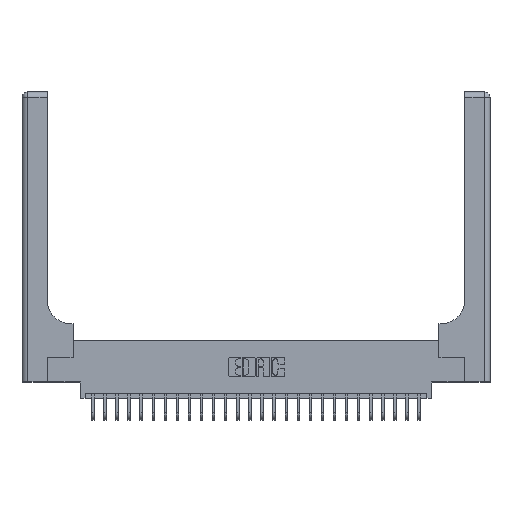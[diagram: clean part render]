
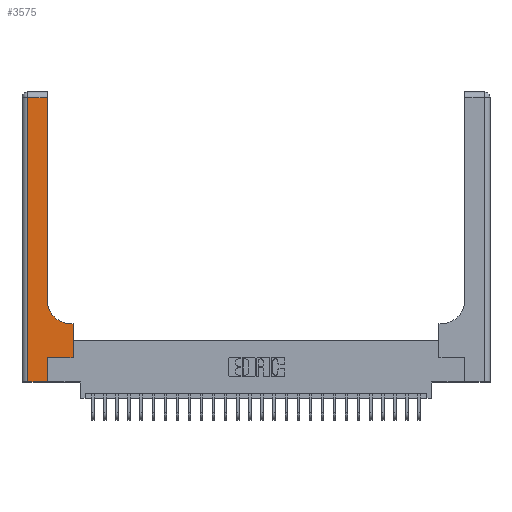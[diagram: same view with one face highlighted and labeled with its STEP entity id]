
A CAD part, top view. The second image highlights one B-rep face of the part: STEP entity #3575.
In plain terms, the highlighted planar face has unit normal (0, 0, 1).
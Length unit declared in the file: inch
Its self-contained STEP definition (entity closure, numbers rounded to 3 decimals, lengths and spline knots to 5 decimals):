
#247 = VERTEX_POINT ( 'NONE', #12926 ) ;
#473 = CARTESIAN_POINT ( 'NONE',  ( 0., 3., 0.37 ) ) ;
#620 = EDGE_CURVE ( 'NONE', #6042, #247, #7801, .T. ) ;
#866 = CARTESIAN_POINT ( 'NONE',  ( 0.06, 0., 0.37 ) ) ;
#962 = DIRECTION ( 'NONE',  ( -1., 0., 0. ) ) ;
#1192 = CARTESIAN_POINT ( 'NONE',  ( 0.265, 0.25, 0.37 ) ) ;
#1237 = EDGE_CURVE ( 'NONE', #19459, #6042, #15908, .T. ) ;
#1306 = DIRECTION ( 'NONE',  ( 0., 1., 0. ) ) ;
#1980 = EDGE_CURVE ( 'NONE', #247, #21757, #3933, .T. ) ;
#2104 = DIRECTION ( 'NONE',  ( -1., 0., 0. ) ) ;
#2456 = CARTESIAN_POINT ( 'NONE',  ( 0., 2.94, 0.37 ) ) ;
#2571 = CARTESIAN_POINT ( 'NONE',  ( 0.528, 0.25, 0.37 ) ) ;
#3368 = CARTESIAN_POINT ( 'NONE',  ( 0.26, 0.85, 0.37 ) ) ;
#3378 = CARTESIAN_POINT ( 'NONE',  ( 0.26, 3., 0.37 ) ) ;
#3511 = ORIENTED_EDGE ( 'NONE', *, *, #12563, .T. ) ;
#3575 = ADVANCED_FACE ( 'NONE', ( #25442 ), #13136, .F. ) ;
#3933 = LINE ( 'NONE', #5241, #25619 ) ;
#4005 = DIRECTION ( 'NONE',  ( 1., 0., 0. ) ) ;
#4239 = LINE ( 'NONE', #24141, #20331 ) ;
#4367 = VECTOR ( 'NONE', #2104, 39.37008 ) ;
#4563 = VERTEX_POINT ( 'NONE', #16521 ) ;
#4620 = CARTESIAN_POINT ( 'NONE',  ( 0.06, 3., 0.37 ) ) ;
#4726 = ORIENTED_EDGE ( 'NONE', *, *, #8363, .T. ) ;
#4866 = DIRECTION ( 'NONE',  ( -1., 0., 0. ) ) ;
#4985 = LINE ( 'NONE', #3378, #26697 ) ;
#5241 = CARTESIAN_POINT ( 'NONE',  ( 0.26, 0.6, 0.37 ) ) ;
#5452 = CIRCLE ( 'NONE', #27289, 0.25 ) ;
#6042 = VERTEX_POINT ( 'NONE', #22230 ) ;
#6170 = EDGE_CURVE ( 'NONE', #21757, #24052, #5452, .T. ) ;
#6517 = CARTESIAN_POINT ( 'NONE',  ( 0.265, 0.25, 0.37 ) ) ;
#7495 = VECTOR ( 'NONE', #4005, 39.37008 ) ;
#7801 = LINE ( 'NONE', #2571, #16007 ) ;
#8273 = ORIENTED_EDGE ( 'NONE', *, *, #1980, .T. ) ;
#8363 = EDGE_CURVE ( 'NONE', #4563, #13589, #18525, .T. ) ;
#8465 = ORIENTED_EDGE ( 'NONE', *, *, #14059, .T. ) ;
#8792 = EDGE_CURVE ( 'NONE', #24052, #4563, #4985, .T. ) ;
#8857 = DIRECTION ( 'NONE',  ( 0., -1., 0. ) ) ;
#9061 = DIRECTION ( 'NONE',  ( 0., 1., 0. ) ) ;
#10220 = ORIENTED_EDGE ( 'NONE', *, *, #8792, .T. ) ;
#10296 = DIRECTION ( 'NONE',  ( 0., 0., -1. ) ) ;
#10834 = EDGE_CURVE ( 'NONE', #15806, #13423, #16705, .T. ) ;
#12563 = EDGE_CURVE ( 'NONE', #13589, #15806, #18481, .T. ) ;
#12926 = CARTESIAN_POINT ( 'NONE',  ( 0.528, 0.6, 0.37 ) ) ;
#13136 = PLANE ( 'NONE',  #20071 ) ;
#13225 = DIRECTION ( 'NONE',  ( 0., 0., -1. ) ) ;
#13303 = ORIENTED_EDGE ( 'NONE', *, *, #6170, .T. ) ;
#13423 = VERTEX_POINT ( 'NONE', #25823 ) ;
#13589 = VERTEX_POINT ( 'NONE', #22096 ) ;
#14059 = EDGE_CURVE ( 'NONE', #13423, #19459, #4239, .T. ) ;
#14183 = ORIENTED_EDGE ( 'NONE', *, *, #1237, .T. ) ;
#14316 = CARTESIAN_POINT ( 'NONE',  ( 0.51, 0.85, 0.37 ) ) ;
#15806 = VERTEX_POINT ( 'NONE', #866 ) ;
#15891 = DIRECTION ( 'NONE',  ( 0., 1., 0. ) ) ;
#15908 = LINE ( 'NONE', #6517, #20874 ) ;
#16007 = VECTOR ( 'NONE', #9061, 39.37008 ) ;
#16521 = CARTESIAN_POINT ( 'NONE',  ( 0.26, 2.94, 0.37 ) ) ;
#16705 = LINE ( 'NONE', #20750, #7495 ) ;
#17126 = ORIENTED_EDGE ( 'NONE', *, *, #10834, .T. ) ;
#18410 = EDGE_LOOP ( 'NONE', ( #10220, #4726, #3511, #17126, #8465, #14183, #25301, #8273, #13303 ) ) ;
#18481 = LINE ( 'NONE', #4620, #25650 ) ;
#18525 = LINE ( 'NONE', #2456, #4367 ) ;
#19459 = VERTEX_POINT ( 'NONE', #1192 ) ;
#20071 = AXIS2_PLACEMENT_3D ( 'NONE', #473, #13225, #4866 ) ;
#20331 = VECTOR ( 'NONE', #1306, 39.37008 ) ;
#20750 = CARTESIAN_POINT ( 'NONE',  ( 0., 0., 0.37 ) ) ;
#20874 = VECTOR ( 'NONE', #27195, 39.37008 ) ;
#21757 = VERTEX_POINT ( 'NONE', #23158 ) ;
#22096 = CARTESIAN_POINT ( 'NONE',  ( 0.06, 2.94, 0.37 ) ) ;
#22230 = CARTESIAN_POINT ( 'NONE',  ( 0.528, 0.25, 0.37 ) ) ;
#23158 = CARTESIAN_POINT ( 'NONE',  ( 0.51, 0.6, 0.37 ) ) ;
#24052 = VERTEX_POINT ( 'NONE', #3368 ) ;
#24141 = CARTESIAN_POINT ( 'NONE',  ( 0.265, 0., 0.37 ) ) ;
#25301 = ORIENTED_EDGE ( 'NONE', *, *, #620, .T. ) ;
#25442 = FACE_OUTER_BOUND ( 'NONE', #18410, .T. ) ;
#25619 = VECTOR ( 'NONE', #962, 39.37008 ) ;
#25650 = VECTOR ( 'NONE', #8857, 39.37008 ) ;
#25823 = CARTESIAN_POINT ( 'NONE',  ( 0.265, 0., 0.37 ) ) ;
#26697 = VECTOR ( 'NONE', #15891, 39.37008 ) ;
#26735 = DIRECTION ( 'NONE',  ( 1., 0., 0. ) ) ;
#27195 = DIRECTION ( 'NONE',  ( 1., 0., 0. ) ) ;
#27289 = AXIS2_PLACEMENT_3D ( 'NONE', #14316, #10296, #26735 ) ;
